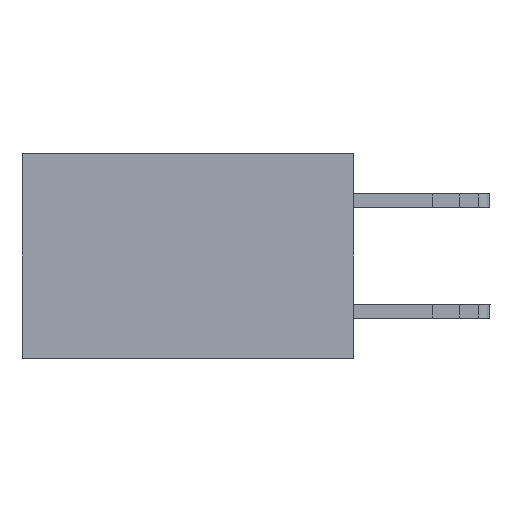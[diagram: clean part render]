
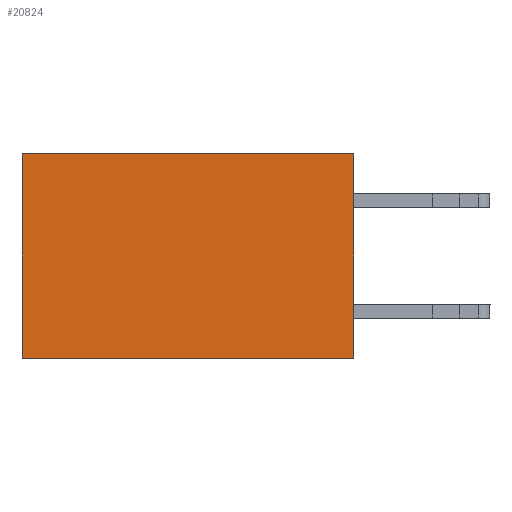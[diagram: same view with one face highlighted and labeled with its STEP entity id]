
A CAD part, left-side view. The second image highlights one B-rep face of the part: STEP entity #20824.
In plain terms, the highlighted planar face has unit normal (-1, 0, 0).
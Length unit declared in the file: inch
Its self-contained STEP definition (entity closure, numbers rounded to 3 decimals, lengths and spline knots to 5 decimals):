
#135 = DIRECTION ( 'NONE',  ( 0., 1., 0. ) ) ;
#577 = ORIENTED_EDGE ( 'NONE', *, *, #12861, .F. ) ;
#837 = VERTEX_POINT ( 'NONE', #1213 ) ;
#1213 = CARTESIAN_POINT ( 'NONE',  ( 0.2875, 0.6, 0. ) ) ;
#1849 = CARTESIAN_POINT ( 'NONE',  ( 0.2875, 0.6, -0.37 ) ) ;
#2011 = CARTESIAN_POINT ( 'NONE',  ( 0.2875, 0., -0.37 ) ) ;
#2359 = LINE ( 'NONE', #10808, #18965 ) ;
#3359 = EDGE_CURVE ( 'NONE', #21485, #9060, #2359, .T. ) ;
#4242 = LINE ( 'NONE', #21252, #17109 ) ;
#6457 = AXIS2_PLACEMENT_3D ( 'NONE', #12743, #12875, #21749 ) ;
#6459 = ORIENTED_EDGE ( 'NONE', *, *, #19555, .T. ) ;
#6630 = FACE_OUTER_BOUND ( 'NONE', #9144, .T. ) ;
#8320 = LINE ( 'NONE', #16811, #25835 ) ;
#9060 = VERTEX_POINT ( 'NONE', #1849 ) ;
#9144 = EDGE_LOOP ( 'NONE', ( #6459, #25532, #577, #24916 ) ) ;
#9511 = VERTEX_POINT ( 'NONE', #14209 ) ;
#10808 = CARTESIAN_POINT ( 'NONE',  ( 0.2875, 0., -0.37 ) ) ;
#10944 = PLANE ( 'NONE',  #6457 ) ;
#11092 = CARTESIAN_POINT ( 'NONE',  ( 0.2875, 0., 0. ) ) ;
#12448 = EDGE_CURVE ( 'NONE', #9511, #837, #8320, .T. ) ;
#12743 = CARTESIAN_POINT ( 'NONE',  ( 0.2875, 0., 0. ) ) ;
#12861 = EDGE_CURVE ( 'NONE', #9511, #21485, #13300, .T. ) ;
#12875 = DIRECTION ( 'NONE',  ( 1., 0., 0. ) ) ;
#13159 = DIRECTION ( 'NONE',  ( 0., 0., -1. ) ) ;
#13300 = LINE ( 'NONE', #11092, #20511 ) ;
#14209 = CARTESIAN_POINT ( 'NONE',  ( 0.2875, 0., 0. ) ) ;
#14737 = DIRECTION ( 'NONE',  ( 0., 1., 0. ) ) ;
#16811 = CARTESIAN_POINT ( 'NONE',  ( 0.2875, 0., 0. ) ) ;
#17109 = VECTOR ( 'NONE', #18499, 39.37008 ) ;
#18499 = DIRECTION ( 'NONE',  ( 0., 0., -1. ) ) ;
#18965 = VECTOR ( 'NONE', #135, 39.37008 ) ;
#19555 = EDGE_CURVE ( 'NONE', #837, #9060, #4242, .T. ) ;
#20511 = VECTOR ( 'NONE', #13159, 39.37008 ) ;
#20824 = ADVANCED_FACE ( 'NONE', ( #6630 ), #10944, .F. ) ;
#21252 = CARTESIAN_POINT ( 'NONE',  ( 0.2875, 0.6, 0. ) ) ;
#21485 = VERTEX_POINT ( 'NONE', #2011 ) ;
#21749 = DIRECTION ( 'NONE',  ( 0., 0., -1. ) ) ;
#24916 = ORIENTED_EDGE ( 'NONE', *, *, #12448, .T. ) ;
#25532 = ORIENTED_EDGE ( 'NONE', *, *, #3359, .F. ) ;
#25835 = VECTOR ( 'NONE', #14737, 39.37008 ) ;
